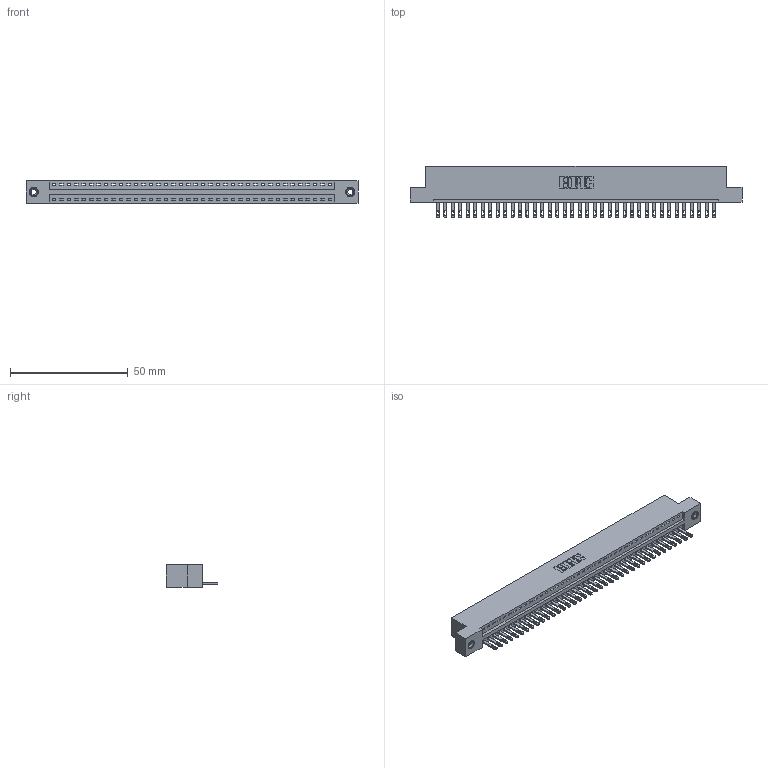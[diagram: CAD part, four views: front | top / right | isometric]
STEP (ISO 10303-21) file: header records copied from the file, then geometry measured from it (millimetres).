
FILE_DESCRIPTION (( 'STEP AP203' ), '1' );
FILE_NAME ('346-038-500-108.STEP', '2018-08-24T04:11:38', ( '' ), ( '' ), 'SwSTEP 2.0', 'SolidWorks 2016', '' );
FILE_SCHEMA (( 'CONFIG_CONTROL_DESIGN' ));
Length unit declared in the file: inch
Products named in the file (4): 346 Part_Flush Mounting Lugs - 0.156 Dia-TI; 345-292-001_345-293-100; 345-250-001_345-250-003-102; 346-038-500-108
Assembly tree (41 placements, depth 2):
  346-038-500-108
    346 Part_Flush Mounting Lugs - 0.156 Dia-TI
    345-292-001_345-293-100  x38
    345-250-001_345-250-003-102  x2
Bounding box: 141.22 x 21.84 x 9.4 mm (x, y, z)
Volume: 13507.7 mm3; surface area: 16950.1 mm2
Topology: 41 solids, 41 shells, 2234 faces, 6849 edges, 4558 vertices
Faces by surface type: plane 1400, cylinder 818, cone 12, torus 4
Entity records: 25238 total; most frequent: CARTESIAN_POINT 4309, ORIENTED_EDGE 4274, DIRECTION 3835, EDGE_CURVE 2137, LINE 1829, VECTOR 1829, VERTEX_POINT 1420, AXIS2_PLACEMENT_3D 1003
